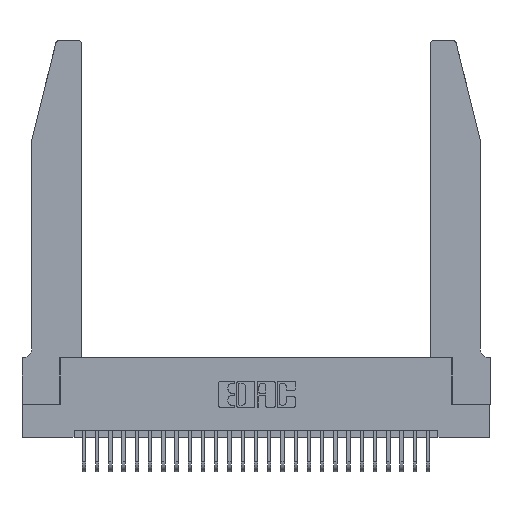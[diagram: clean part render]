
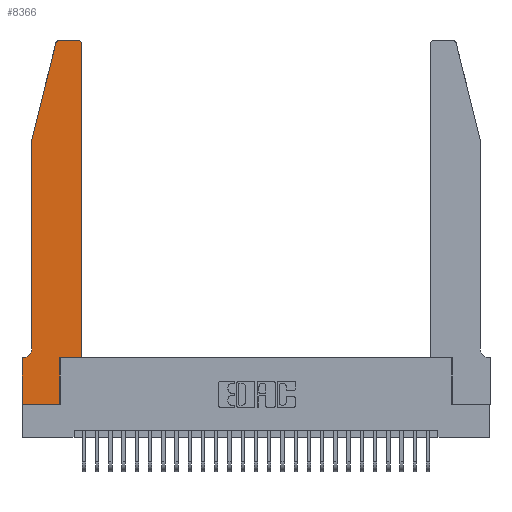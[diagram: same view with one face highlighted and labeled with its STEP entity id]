
A CAD part, top view. The second image highlights one B-rep face of the part: STEP entity #8366.
In plain terms, the highlighted planar face has unit normal (0, 0, 1).
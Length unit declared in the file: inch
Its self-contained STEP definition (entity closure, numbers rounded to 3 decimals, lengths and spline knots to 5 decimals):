
#4 = DIRECTION ( 'NONE',  ( 0., 0., -1. ) ) ;
#412 = VERTEX_POINT ( 'NONE', #5810 ) ;
#425 = ORIENTED_EDGE ( 'NONE', *, *, #16088, .T. ) ;
#532 = ORIENTED_EDGE ( 'NONE', *, *, #18438, .T. ) ;
#820 = CARTESIAN_POINT ( 'NONE',  ( 0.2865, 0.35, 0.37 ) ) ;
#1148 = EDGE_CURVE ( 'NONE', #10484, #21612, #11140, .T. ) ;
#1198 = DIRECTION ( 'NONE',  ( 1., 0., 0. ) ) ;
#1205 = CARTESIAN_POINT ( 'NONE',  ( 0.4205, 2.75, 0.37 ) ) ;
#1651 = ORIENTED_EDGE ( 'NONE', *, *, #3955, .T. ) ;
#1804 = ORIENTED_EDGE ( 'NONE', *, *, #1148, .T. ) ;
#2649 = CARTESIAN_POINT ( 'NONE',  ( 0.0755, 0.35, 0.37 ) ) ;
#2661 = ORIENTED_EDGE ( 'NONE', *, *, #3100, .T. ) ;
#3100 = EDGE_CURVE ( 'NONE', #10377, #3533, #4127, .T. ) ;
#3533 = VERTEX_POINT ( 'NONE', #9501 ) ;
#3552 = DIRECTION ( 'NONE',  ( 0., 1., 0. ) ) ;
#3706 = CARTESIAN_POINT ( 'NONE',  ( 0.25487, 2.72718, 0.37 ) ) ;
#3839 = CIRCLE ( 'NONE', #5611, 0.07 ) ;
#3955 = EDGE_CURVE ( 'NONE', #3533, #412, #16582, .T. ) ;
#4127 = LINE ( 'NONE', #19846, #14656 ) ;
#5425 = DIRECTION ( 'NONE',  ( 0., -1., 0. ) ) ;
#5483 = EDGE_CURVE ( 'NONE', #7470, #9380, #24290, .T. ) ;
#5611 = AXIS2_PLACEMENT_3D ( 'NONE', #12745, #4, #14870 ) ;
#5810 = CARTESIAN_POINT ( 'NONE',  ( 0.4505, 2.72, 0.37 ) ) ;
#6647 = CARTESIAN_POINT ( 'NONE',  ( 0., 0.35, 0.37 ) ) ;
#6706 = DIRECTION ( 'NONE',  ( 0., 0., 1. ) ) ;
#6972 = CIRCLE ( 'NONE', #9239, 0.03 ) ;
#7196 = LINE ( 'NONE', #12595, #11418 ) ;
#7458 = DIRECTION ( 'NONE',  ( -0.239, -0.971, 0. ) ) ;
#7470 = VERTEX_POINT ( 'NONE', #3706 ) ;
#7661 = EDGE_CURVE ( 'NONE', #9380, #24627, #20776, .T. ) ;
#7731 = LINE ( 'NONE', #22237, #23091 ) ;
#7943 = CARTESIAN_POINT ( 'NONE',  ( 0., 0.35, 0.37 ) ) ;
#8366 = ADVANCED_FACE ( 'NONE', ( #15496 ), #23365, .T. ) ;
#8465 = CARTESIAN_POINT ( 'NONE',  ( 0.2605, 2.75, 0.37 ) ) ;
#9239 = AXIS2_PLACEMENT_3D ( 'NONE', #26299, #13878, #1198 ) ;
#9380 = VERTEX_POINT ( 'NONE', #22725 ) ;
#9501 = CARTESIAN_POINT ( 'NONE',  ( 0.4505, 0.35, 0.37 ) ) ;
#10283 = ORIENTED_EDGE ( 'NONE', *, *, #16388, .T. ) ;
#10377 = VERTEX_POINT ( 'NONE', #820 ) ;
#10484 = VERTEX_POINT ( 'NONE', #1205 ) ;
#10510 = VECTOR ( 'NONE', #23063, 39.37008 ) ;
#10609 = EDGE_CURVE ( 'NONE', #16960, #11431, #7196, .T. ) ;
#10839 = DIRECTION ( 'NONE',  ( 0., 0., 1. ) ) ;
#11140 = LINE ( 'NONE', #8465, #10510 ) ;
#11418 = VECTOR ( 'NONE', #14730, 39.37008 ) ;
#11431 = VERTEX_POINT ( 'NONE', #25735 ) ;
#12595 = CARTESIAN_POINT ( 'NONE',  ( 0., 0., 0.37 ) ) ;
#12745 = CARTESIAN_POINT ( 'NONE',  ( 0.0055, 0.42, 0.37 ) ) ;
#13240 = VECTOR ( 'NONE', #17401, 39.37008 ) ;
#13335 = LINE ( 'NONE', #26442, #23809 ) ;
#13807 = CARTESIAN_POINT ( 'NONE',  ( 0., 0., 0.37 ) ) ;
#13878 = DIRECTION ( 'NONE',  ( 0., 0., 1. ) ) ;
#14182 = VERTEX_POINT ( 'NONE', #25601 ) ;
#14471 = LINE ( 'NONE', #2649, #13240 ) ;
#14656 = VECTOR ( 'NONE', #21962, 39.37008 ) ;
#14730 = DIRECTION ( 'NONE',  ( 1., 0., 0. ) ) ;
#14736 = CARTESIAN_POINT ( 'NONE',  ( 0.0755, 2., 0.37 ) ) ;
#14864 = CARTESIAN_POINT ( 'NONE',  ( 0.4505, 0.35, 0.37 ) ) ;
#14870 = DIRECTION ( 'NONE',  ( -1., 0., 0. ) ) ;
#15064 = ORIENTED_EDGE ( 'NONE', *, *, #16716, .T. ) ;
#15496 = FACE_OUTER_BOUND ( 'NONE', #23760, .T. ) ;
#15773 = CARTESIAN_POINT ( 'NONE',  ( 0.0755, 2., 0.37 ) ) ;
#16088 = EDGE_CURVE ( 'NONE', #24627, #14182, #3839, .T. ) ;
#16323 = CARTESIAN_POINT ( 'NONE',  ( 0.284, 2.75, 0.37 ) ) ;
#16388 = EDGE_CURVE ( 'NONE', #11431, #10377, #13335, .T. ) ;
#16582 = LINE ( 'NONE', #14864, #26902 ) ;
#16637 = CIRCLE ( 'NONE', #24645, 0.03 ) ;
#16716 = EDGE_CURVE ( 'NONE', #21612, #7470, #16637, .T. ) ;
#16960 = VERTEX_POINT ( 'NONE', #13807 ) ;
#16983 = DIRECTION ( 'NONE',  ( 0., 1., 0. ) ) ;
#17401 = DIRECTION ( 'NONE',  ( -1., 0., 0. ) ) ;
#17561 = ORIENTED_EDGE ( 'NONE', *, *, #18848, .T. ) ;
#17715 = ORIENTED_EDGE ( 'NONE', *, *, #5483, .T. ) ;
#18438 = EDGE_CURVE ( 'NONE', #25446, #16960, #7731, .T. ) ;
#18848 = EDGE_CURVE ( 'NONE', #14182, #25446, #14471, .T. ) ;
#19226 = CARTESIAN_POINT ( 'NONE',  ( 0.284, 2.72, 0.37 ) ) ;
#19846 = CARTESIAN_POINT ( 'NONE',  ( 0.4505, 0.35, 0.37 ) ) ;
#20116 = VECTOR ( 'NONE', #21038, 39.37008 ) ;
#20776 = LINE ( 'NONE', #14736, #20116 ) ;
#21038 = DIRECTION ( 'NONE',  ( 0., -1., 0. ) ) ;
#21334 = DIRECTION ( 'NONE',  ( 1., 0., 0. ) ) ;
#21612 = VERTEX_POINT ( 'NONE', #16323 ) ;
#21756 = ORIENTED_EDGE ( 'NONE', *, *, #26801, .T. ) ;
#21962 = DIRECTION ( 'NONE',  ( 1., 0., 0. ) ) ;
#22237 = CARTESIAN_POINT ( 'NONE',  ( 0., 0., 0.37 ) ) ;
#22725 = CARTESIAN_POINT ( 'NONE',  ( 0.0755, 2., 0.37 ) ) ;
#23063 = DIRECTION ( 'NONE',  ( -1., 0., 0. ) ) ;
#23091 = VECTOR ( 'NONE', #5425, 39.37008 ) ;
#23365 = PLANE ( 'NONE',  #25034 ) ;
#23632 = ORIENTED_EDGE ( 'NONE', *, *, #10609, .T. ) ;
#23657 = VECTOR ( 'NONE', #7458, 39.37008 ) ;
#23760 = EDGE_LOOP ( 'NONE', ( #1804, #15064, #17715, #25302, #425, #17561, #532, #23632, #10283, #2661, #1651, #21756 ) ) ;
#23809 = VECTOR ( 'NONE', #3552, 39.37008 ) ;
#24290 = LINE ( 'NONE', #15773, #23657 ) ;
#24627 = VERTEX_POINT ( 'NONE', #26140 ) ;
#24645 = AXIS2_PLACEMENT_3D ( 'NONE', #19226, #6706, #21334 ) ;
#25034 = AXIS2_PLACEMENT_3D ( 'NONE', #6647, #10839, #25384 ) ;
#25302 = ORIENTED_EDGE ( 'NONE', *, *, #7661, .T. ) ;
#25384 = DIRECTION ( 'NONE',  ( 1., 0., 0. ) ) ;
#25446 = VERTEX_POINT ( 'NONE', #7943 ) ;
#25601 = CARTESIAN_POINT ( 'NONE',  ( 0.0055, 0.35, 0.37 ) ) ;
#25735 = CARTESIAN_POINT ( 'NONE',  ( 0.2865, 0., 0.37 ) ) ;
#26140 = CARTESIAN_POINT ( 'NONE',  ( 0.0755, 0.42, 0.37 ) ) ;
#26299 = CARTESIAN_POINT ( 'NONE',  ( 0.4205, 2.72, 0.37 ) ) ;
#26442 = CARTESIAN_POINT ( 'NONE',  ( 0.2865, 0.35, 0.37 ) ) ;
#26801 = EDGE_CURVE ( 'NONE', #412, #10484, #6972, .T. ) ;
#26902 = VECTOR ( 'NONE', #16983, 39.37008 ) ;
